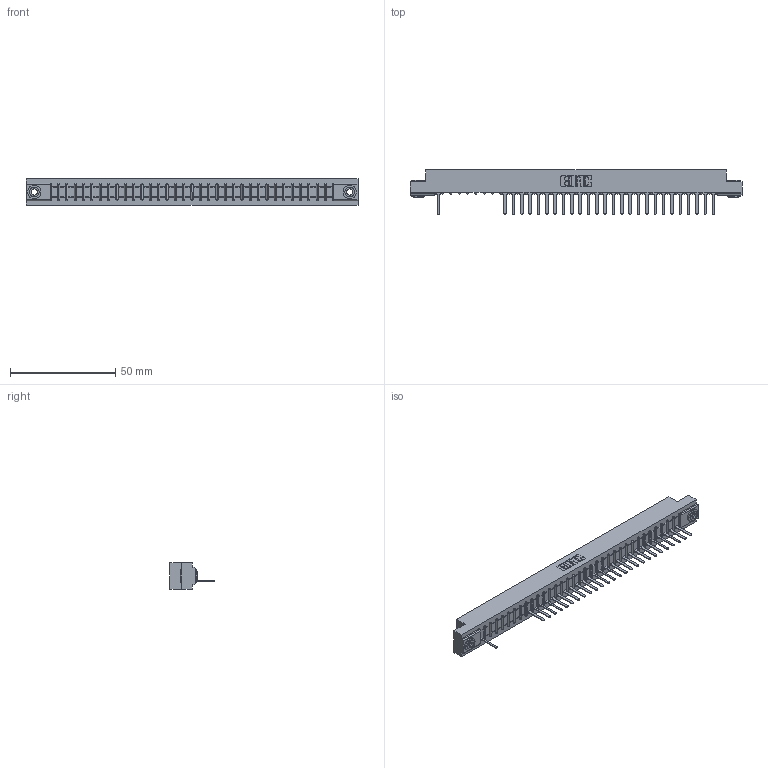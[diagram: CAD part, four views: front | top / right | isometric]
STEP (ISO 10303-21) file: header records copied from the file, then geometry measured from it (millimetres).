
FILE_DESCRIPTION (( 'STEP AP203' ), '1' );
FILE_NAME ('307-034-527-103.STEP', '2018-08-05T00:26:36', ( '' ), ( '' ), 'SwSTEP 2.0', 'SolidWorks 2016', '' );
FILE_SCHEMA (( 'CONFIG_CONTROL_DESIGN' ));
Length unit declared in the file: inch
Products named in the file (4): 307 Part_.156 Dia Mounting Holes; 307-290-001_527; 345-250-002_345-250-002-102; 307-034-527-103
Assembly tree (30 placements, depth 2):
  307-034-527-103
    307 Part_.156 Dia Mounting Holes
    307-290-001_527  x27
    345-250-002_345-250-002-102  x2
Bounding box: 157.73 x 21.11 x 12.7 mm (x, y, z)
Volume: 16246.3 mm3; surface area: 16784.6 mm2
Topology: 30 solids, 30 shells, 1857 faces, 5257 edges, 3370 vertices
Faces by surface type: plane 1177, cylinder 602, sphere 70, cone 8
Entity records: 30943 total; most frequent: CARTESIAN_POINT 5218, ORIENTED_EDGE 5202, DIRECTION 5087, EDGE_CURVE 2601, LINE 1985, VECTOR 1985, VERTEX_POINT 1682, AXIS2_PLACEMENT_3D 1551
